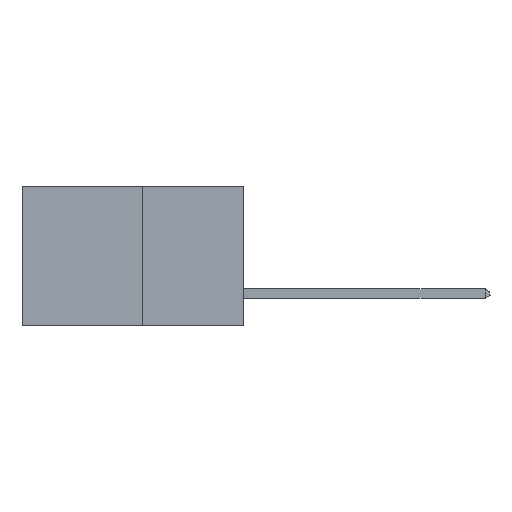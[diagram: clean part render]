
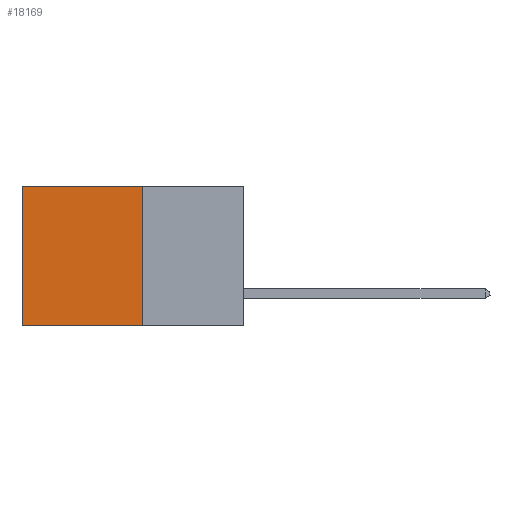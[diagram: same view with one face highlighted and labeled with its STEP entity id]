
A CAD part, left-side view. The second image highlights one B-rep face of the part: STEP entity #18169.
In plain terms, the highlighted planar face has unit normal (-1, 0, 0).
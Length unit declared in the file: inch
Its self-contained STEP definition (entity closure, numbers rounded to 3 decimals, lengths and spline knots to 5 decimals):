
#837 = VECTOR ( 'NONE', #6168, 39.37008 ) ;
#2212 = ORIENTED_EDGE ( 'NONE', *, *, #11681, .T. ) ;
#3265 = CARTESIAN_POINT ( 'NONE',  ( 0.277, 0.27, -0.37 ) ) ;
#4632 = EDGE_CURVE ( 'NONE', #12014, #10422, #22382, .T. ) ;
#4710 = DIRECTION ( 'NONE',  ( 0., 0., -1. ) ) ;
#5203 = DIRECTION ( 'NONE',  ( 0., 0., -1. ) ) ;
#6168 = DIRECTION ( 'NONE',  ( 0., 1., 0. ) ) ;
#6255 = VERTEX_POINT ( 'NONE', #14629 ) ;
#7028 = CARTESIAN_POINT ( 'NONE',  ( 0.277, 0.59, -0.37 ) ) ;
#7483 = VECTOR ( 'NONE', #22199, 39.37008 ) ;
#8227 = DIRECTION ( 'NONE',  ( 0., 1., 0. ) ) ;
#10112 = CARTESIAN_POINT ( 'NONE',  ( 0.277, 0.27, 0. ) ) ;
#10371 = LINE ( 'NONE', #17432, #837 ) ;
#10422 = VERTEX_POINT ( 'NONE', #17741 ) ;
#11681 = EDGE_CURVE ( 'NONE', #6255, #18140, #18513, .T. ) ;
#12014 = VERTEX_POINT ( 'NONE', #10112 ) ;
#13611 = VECTOR ( 'NONE', #8227, 39.37008 ) ;
#14563 = ORIENTED_EDGE ( 'NONE', *, *, #16079, .T. ) ;
#14616 = PLANE ( 'NONE',  #21450 ) ;
#14629 = CARTESIAN_POINT ( 'NONE',  ( 0.277, 0.59, 0. ) ) ;
#16000 = EDGE_CURVE ( 'NONE', #10422, #18140, #10371, .T. ) ;
#16079 = EDGE_CURVE ( 'NONE', #12014, #6255, #18571, .T. ) ;
#16482 = DIRECTION ( 'NONE',  ( 1., 0., 0. ) ) ;
#16628 = CARTESIAN_POINT ( 'NONE',  ( 0.277, 0.27, -0.37 ) ) ;
#17432 = CARTESIAN_POINT ( 'NONE',  ( 0.277, 0.27, -0.37 ) ) ;
#17741 = CARTESIAN_POINT ( 'NONE',  ( 0.277, 0.27, -0.37 ) ) ;
#17916 = VECTOR ( 'NONE', #4710, 39.37008 ) ;
#18140 = VERTEX_POINT ( 'NONE', #7028 ) ;
#18169 = ADVANCED_FACE ( 'NONE', ( #22820 ), #14616, .F. ) ;
#18513 = LINE ( 'NONE', #23366, #17916 ) ;
#18571 = LINE ( 'NONE', #23179, #13611 ) ;
#20499 = EDGE_LOOP ( 'NONE', ( #2212, #23670, #20643, #14563 ) ) ;
#20643 = ORIENTED_EDGE ( 'NONE', *, *, #4632, .F. ) ;
#21450 = AXIS2_PLACEMENT_3D ( 'NONE', #3265, #16482, #5203 ) ;
#22199 = DIRECTION ( 'NONE',  ( 0., 0., -1. ) ) ;
#22382 = LINE ( 'NONE', #16628, #7483 ) ;
#22820 = FACE_OUTER_BOUND ( 'NONE', #20499, .T. ) ;
#23179 = CARTESIAN_POINT ( 'NONE',  ( 0.277, 0.27, 0. ) ) ;
#23366 = CARTESIAN_POINT ( 'NONE',  ( 0.277, 0.59, -0.37 ) ) ;
#23670 = ORIENTED_EDGE ( 'NONE', *, *, #16000, .F. ) ;
